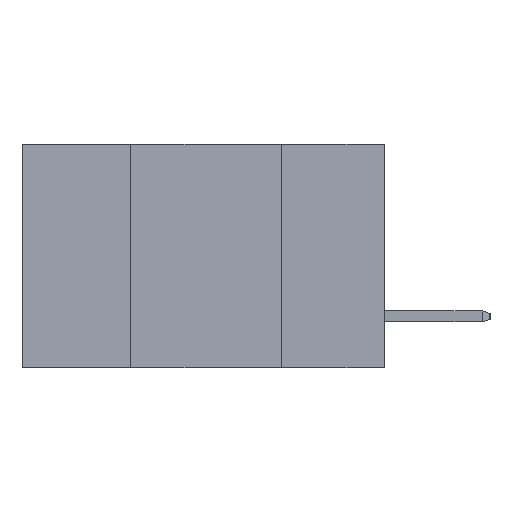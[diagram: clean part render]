
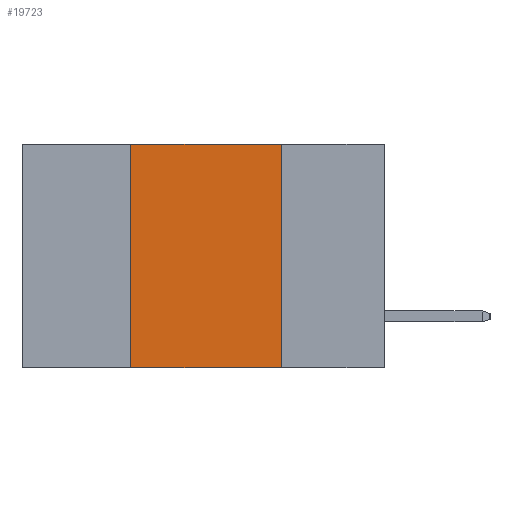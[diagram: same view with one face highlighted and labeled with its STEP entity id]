
A CAD part, left-side view. The second image highlights one B-rep face of the part: STEP entity #19723.
In plain terms, the highlighted planar face has unit normal (-1, 0, 0).
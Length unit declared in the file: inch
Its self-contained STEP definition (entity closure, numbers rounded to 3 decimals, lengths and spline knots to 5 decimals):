
#246 = CARTESIAN_POINT ( 'NONE',  ( 0., 0.42, -0.37 ) ) ;
#1671 = LINE ( 'NONE', #5171, #10610 ) ;
#2113 = EDGE_LOOP ( 'NONE', ( #3786, #8603, #18240, #15407 ) ) ;
#2115 = VERTEX_POINT ( 'NONE', #15206 ) ;
#2773 = LINE ( 'NONE', #19662, #7049 ) ;
#3002 = EDGE_CURVE ( 'NONE', #2115, #13808, #13557, .T. ) ;
#3014 = CARTESIAN_POINT ( 'NONE',  ( 0., 0.6, 0. ) ) ;
#3786 = ORIENTED_EDGE ( 'NONE', *, *, #14922, .F. ) ;
#4841 = PLANE ( 'NONE',  #11842 ) ;
#5171 = CARTESIAN_POINT ( 'NONE',  ( 0., 0.17, -0.37 ) ) ;
#5319 = CARTESIAN_POINT ( 'NONE',  ( 0., 0.17, 0. ) ) ;
#5447 = EDGE_CURVE ( 'NONE', #2115, #14957, #8486, .T. ) ;
#6682 = DIRECTION ( 'NONE',  ( 0., 0., -1. ) ) ;
#7002 = DIRECTION ( 'NONE',  ( 0., 0., -1. ) ) ;
#7049 = VECTOR ( 'NONE', #19682, 39.37008 ) ;
#7889 = VERTEX_POINT ( 'NONE', #5319 ) ;
#8005 = FACE_OUTER_BOUND ( 'NONE', #2113, .T. ) ;
#8486 = LINE ( 'NONE', #246, #16087 ) ;
#8603 = ORIENTED_EDGE ( 'NONE', *, *, #9081, .F. ) ;
#9081 = EDGE_CURVE ( 'NONE', #14957, #7889, #2773, .T. ) ;
#9440 = VECTOR ( 'NONE', #20150, 39.37008 ) ;
#10610 = VECTOR ( 'NONE', #7002, 39.37008 ) ;
#11842 = AXIS2_PLACEMENT_3D ( 'NONE', #3014, #17059, #6682 ) ;
#12456 = CARTESIAN_POINT ( 'NONE',  ( 0., 0.42, 0. ) ) ;
#12879 = CARTESIAN_POINT ( 'NONE',  ( 0., 0.17, -0.37 ) ) ;
#13557 = LINE ( 'NONE', #19574, #9440 ) ;
#13808 = VERTEX_POINT ( 'NONE', #12879 ) ;
#14922 = EDGE_CURVE ( 'NONE', #7889, #13808, #1671, .T. ) ;
#14957 = VERTEX_POINT ( 'NONE', #12456 ) ;
#15206 = CARTESIAN_POINT ( 'NONE',  ( 0., 0.42, -0.37 ) ) ;
#15407 = ORIENTED_EDGE ( 'NONE', *, *, #3002, .T. ) ;
#16087 = VECTOR ( 'NONE', #21866, 39.37008 ) ;
#17059 = DIRECTION ( 'NONE',  ( 1., 0., 0. ) ) ;
#18240 = ORIENTED_EDGE ( 'NONE', *, *, #5447, .F. ) ;
#19574 = CARTESIAN_POINT ( 'NONE',  ( 0., 0.6, -0.37 ) ) ;
#19662 = CARTESIAN_POINT ( 'NONE',  ( 0., 0.6, 0. ) ) ;
#19682 = DIRECTION ( 'NONE',  ( 0., -1., 0. ) ) ;
#19723 = ADVANCED_FACE ( 'NONE', ( #8005 ), #4841, .F. ) ;
#20150 = DIRECTION ( 'NONE',  ( 0., -1., 0. ) ) ;
#21866 = DIRECTION ( 'NONE',  ( 0., 0., 1. ) ) ;
